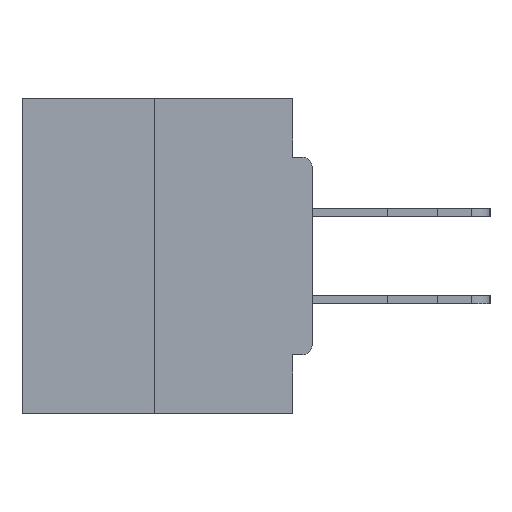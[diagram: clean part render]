
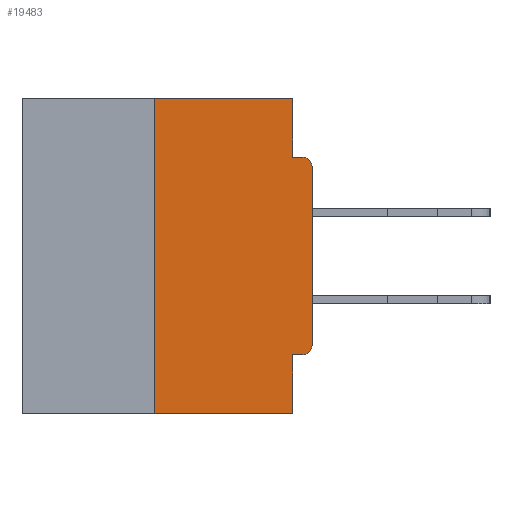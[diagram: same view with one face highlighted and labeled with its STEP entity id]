
A CAD part, left-side view. The second image highlights one B-rep face of the part: STEP entity #19483.
In plain terms, the highlighted planar face has unit normal (-1, 0, 0).
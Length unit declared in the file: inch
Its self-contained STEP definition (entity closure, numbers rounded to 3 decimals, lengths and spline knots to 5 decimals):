
#80 = ORIENTED_EDGE ( 'NONE', *, *, #1926, .T. ) ;
#256 = DIRECTION ( 'NONE',  ( 0., -1., 0. ) ) ;
#749 = DIRECTION ( 'NONE',  ( 0., -1., 0. ) ) ;
#914 = VECTOR ( 'NONE', #256, 39.37008 ) ;
#1011 = DIRECTION ( 'NONE',  ( 0., 0., -1. ) ) ;
#1612 = ORIENTED_EDGE ( 'NONE', *, *, #6984, .F. ) ;
#1926 = EDGE_CURVE ( 'NONE', #32950, #18274, #32608, .T. ) ;
#2175 = VECTOR ( 'NONE', #9857, 39.37008 ) ;
#2617 = CARTESIAN_POINT ( 'NONE',  ( 0., 0.46, -0.5 ) ) ;
#2725 = EDGE_CURVE ( 'NONE', #15768, #28666, #5856, .T. ) ;
#4166 = VERTEX_POINT ( 'NONE', #25600 ) ;
#4204 = CARTESIAN_POINT ( 'NONE',  ( 0., 0.25, 0. ) ) ;
#4969 = EDGE_CURVE ( 'NONE', #28666, #12487, #9104, .T. ) ;
#5028 = CARTESIAN_POINT ( 'NONE',  ( 0., 0.015, -0.0935 ) ) ;
#5075 = AXIS2_PLACEMENT_3D ( 'NONE', #9282, #11765, #30541 ) ;
#5856 = LINE ( 'NONE', #6938, #31682 ) ;
#6159 = CARTESIAN_POINT ( 'NONE',  ( 0., 0.46, 0. ) ) ;
#6243 = ORIENTED_EDGE ( 'NONE', *, *, #7146, .F. ) ;
#6697 = VERTEX_POINT ( 'NONE', #29152 ) ;
#6938 = CARTESIAN_POINT ( 'NONE',  ( 0., 0., -0.4065 ) ) ;
#6984 = EDGE_CURVE ( 'NONE', #22677, #28646, #33994, .T. ) ;
#7146 = EDGE_CURVE ( 'NONE', #6697, #24037, #14261, .T. ) ;
#9104 = LINE ( 'NONE', #33517, #16265 ) ;
#9175 = DIRECTION ( 'NONE',  ( -1., 0., 0. ) ) ;
#9282 = CARTESIAN_POINT ( 'NONE',  ( 0., 0.015, -0.3915 ) ) ;
#9384 = LINE ( 'NONE', #4204, #2175 ) ;
#9644 = DIRECTION ( 'NONE',  ( 0., 0., 1. ) ) ;
#9672 = EDGE_CURVE ( 'NONE', #15768, #32950, #21681, .T. ) ;
#9717 = EDGE_CURVE ( 'NONE', #4166, #22677, #9384, .T. ) ;
#9857 = DIRECTION ( 'NONE',  ( 0., 0., 1. ) ) ;
#10178 = DIRECTION ( 'NONE',  ( 0., 0., -1. ) ) ;
#10929 = CARTESIAN_POINT ( 'NONE',  ( 0., 0.46, 0. ) ) ;
#11335 = DIRECTION ( 'NONE',  ( 0., 0., -1. ) ) ;
#11510 = CARTESIAN_POINT ( 'NONE',  ( 0., 0., -0.0935 ) ) ;
#11538 = CARTESIAN_POINT ( 'NONE',  ( 0., 0.015, -0.1085 ) ) ;
#11765 = DIRECTION ( 'NONE',  ( -1., 0., 0. ) ) ;
#12085 = CARTESIAN_POINT ( 'NONE',  ( 0., 0.25, 0. ) ) ;
#12487 = VERTEX_POINT ( 'NONE', #19181 ) ;
#12519 = CARTESIAN_POINT ( 'NONE',  ( 0., 0., -0.1085 ) ) ;
#12979 = VECTOR ( 'NONE', #749, 39.37008 ) ;
#13151 = LINE ( 'NONE', #29164, #16560 ) ;
#13345 = CARTESIAN_POINT ( 'NONE',  ( 0., 0.031, -0.4065 ) ) ;
#13367 = VECTOR ( 'NONE', #24524, 39.37008 ) ;
#13833 = CARTESIAN_POINT ( 'NONE',  ( 0., 0.015, -0.4065 ) ) ;
#14085 = FACE_OUTER_BOUND ( 'NONE', #33231, .T. ) ;
#14261 = LINE ( 'NONE', #11510, #12979 ) ;
#14350 = VECTOR ( 'NONE', #9644, 39.37008 ) ;
#14562 = ORIENTED_EDGE ( 'NONE', *, *, #4969, .F. ) ;
#14638 = AXIS2_PLACEMENT_3D ( 'NONE', #11538, #9175, #1011 ) ;
#15171 = CARTESIAN_POINT ( 'NONE',  ( 0., 0., 0. ) ) ;
#15768 = VERTEX_POINT ( 'NONE', #13833 ) ;
#16265 = VECTOR ( 'NONE', #25441, 39.37008 ) ;
#16301 = CARTESIAN_POINT ( 'NONE',  ( 0., 0.031, 0. ) ) ;
#16560 = VECTOR ( 'NONE', #10178, 39.37008 ) ;
#17125 = DIRECTION ( 'NONE',  ( 1., 0., 0. ) ) ;
#18274 = VERTEX_POINT ( 'NONE', #12519 ) ;
#19181 = CARTESIAN_POINT ( 'NONE',  ( 0., 0.031, -0.5 ) ) ;
#19483 = ADVANCED_FACE ( 'NONE', ( #14085 ), #22611, .F. ) ;
#20094 = EDGE_CURVE ( 'NONE', #18274, #24037, #28212, .T. ) ;
#21681 = CIRCLE ( 'NONE', #5075, 0.015 ) ;
#22611 = PLANE ( 'NONE',  #28759 ) ;
#22677 = VERTEX_POINT ( 'NONE', #12085 ) ;
#22720 = ORIENTED_EDGE ( 'NONE', *, *, #30285, .F. ) ;
#23647 = ORIENTED_EDGE ( 'NONE', *, *, #26629, .T. ) ;
#24037 = VERTEX_POINT ( 'NONE', #5028 ) ;
#24095 = ORIENTED_EDGE ( 'NONE', *, *, #9672, .T. ) ;
#24524 = DIRECTION ( 'NONE',  ( 0., -1., 0. ) ) ;
#25441 = DIRECTION ( 'NONE',  ( 0., 0., -1. ) ) ;
#25600 = CARTESIAN_POINT ( 'NONE',  ( 0., 0.25, -0.5 ) ) ;
#25879 = DIRECTION ( 'NONE',  ( 0., 1., 0. ) ) ;
#26456 = CARTESIAN_POINT ( 'NONE',  ( 0., 0., -0.3915 ) ) ;
#26629 = EDGE_CURVE ( 'NONE', #4166, #12487, #28684, .T. ) ;
#28212 = CIRCLE ( 'NONE', #14638, 0.015 ) ;
#28646 = VERTEX_POINT ( 'NONE', #16301 ) ;
#28666 = VERTEX_POINT ( 'NONE', #13345 ) ;
#28684 = LINE ( 'NONE', #2617, #13367 ) ;
#28759 = AXIS2_PLACEMENT_3D ( 'NONE', #6159, #17125, #11335 ) ;
#29152 = CARTESIAN_POINT ( 'NONE',  ( 0., 0.031, -0.0935 ) ) ;
#29164 = CARTESIAN_POINT ( 'NONE',  ( 0., 0.031, 0. ) ) ;
#30285 = EDGE_CURVE ( 'NONE', #28646, #6697, #13151, .T. ) ;
#30541 = DIRECTION ( 'NONE',  ( 0., 0., -1. ) ) ;
#31682 = VECTOR ( 'NONE', #25879, 39.37008 ) ;
#31885 = ORIENTED_EDGE ( 'NONE', *, *, #20094, .T. ) ;
#32608 = LINE ( 'NONE', #15171, #14350 ) ;
#32950 = VERTEX_POINT ( 'NONE', #26456 ) ;
#33231 = EDGE_LOOP ( 'NONE', ( #1612, #33471, #23647, #14562, #34228, #24095, #80, #31885, #6243, #22720 ) ) ;
#33471 = ORIENTED_EDGE ( 'NONE', *, *, #9717, .F. ) ;
#33517 = CARTESIAN_POINT ( 'NONE',  ( 0., 0.031, -0.5 ) ) ;
#33994 = LINE ( 'NONE', #10929, #914 ) ;
#34228 = ORIENTED_EDGE ( 'NONE', *, *, #2725, .F. ) ;
